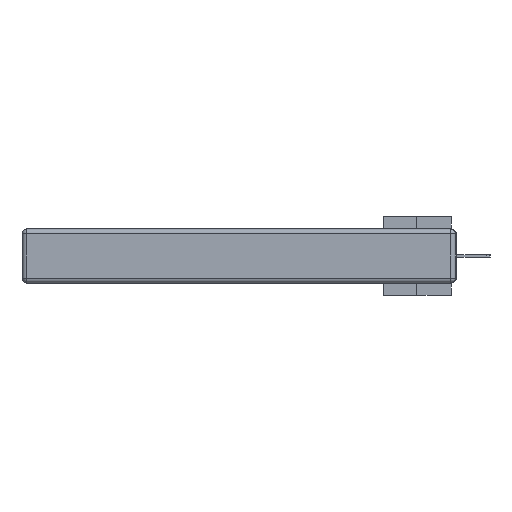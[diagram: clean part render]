
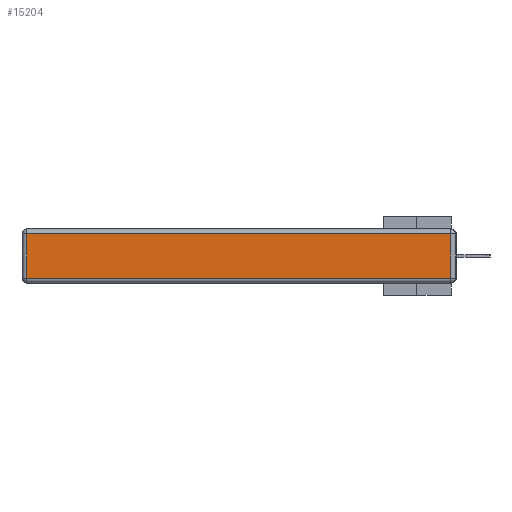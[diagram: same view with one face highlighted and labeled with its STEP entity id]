
A CAD part, left-side view. The second image highlights one B-rep face of the part: STEP entity #15204.
In plain terms, the highlighted planar face has unit normal (-1, 0, 0).
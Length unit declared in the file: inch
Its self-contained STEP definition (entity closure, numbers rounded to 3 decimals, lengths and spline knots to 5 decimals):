
#1295 = DIRECTION ( 'NONE',  ( 0., 0., 1. ) ) ;
#2085 = EDGE_CURVE ( 'NONE', #8228, #25494, #31816, .T. ) ;
#2964 = EDGE_LOOP ( 'NONE', ( #28196, #27298, #23899, #24399 ) ) ;
#3257 = EDGE_CURVE ( 'NONE', #29479, #37648, #40061, .T. ) ;
#3329 = EDGE_CURVE ( 'NONE', #37648, #8228, #33563, .T. ) ;
#4023 = DIRECTION ( 'NONE',  ( 0., 1., 0. ) ) ;
#6081 = EDGE_CURVE ( 'NONE', #25494, #29479, #33803, .T. ) ;
#7036 = VECTOR ( 'NONE', #8781, 39.37008 ) ;
#8228 = VERTEX_POINT ( 'NONE', #17360 ) ;
#8781 = DIRECTION ( 'NONE',  ( 0., 0., -1. ) ) ;
#9344 = VECTOR ( 'NONE', #4023, 39.37008 ) ;
#14401 = DIRECTION ( 'NONE',  ( 0., 0., 1. ) ) ;
#14841 = AXIS2_PLACEMENT_3D ( 'NONE', #17502, #24609, #1295 ) ;
#15038 = CARTESIAN_POINT ( 'NONE',  ( 0., 2.72, -0.343 ) ) ;
#15204 = ADVANCED_FACE ( 'NONE', ( #24806 ), #34475, .T. ) ;
#17360 = CARTESIAN_POINT ( 'NONE',  ( 0., 2.72, -0.03 ) ) ;
#17502 = CARTESIAN_POINT ( 'NONE',  ( 0., 0., -0.343 ) ) ;
#21053 = VECTOR ( 'NONE', #14401, 39.37008 ) ;
#22608 = CARTESIAN_POINT ( 'NONE',  ( 0., 0.03, -0.313 ) ) ;
#23899 = ORIENTED_EDGE ( 'NONE', *, *, #3329, .T. ) ;
#24399 = ORIENTED_EDGE ( 'NONE', *, *, #2085, .T. ) ;
#24609 = DIRECTION ( 'NONE',  ( -1., 0., 0. ) ) ;
#24806 = FACE_OUTER_BOUND ( 'NONE', #2964, .T. ) ;
#25494 = VERTEX_POINT ( 'NONE', #38235 ) ;
#25695 = VECTOR ( 'NONE', #34245, 39.37008 ) ;
#27298 = ORIENTED_EDGE ( 'NONE', *, *, #3257, .T. ) ;
#28196 = ORIENTED_EDGE ( 'NONE', *, *, #6081, .T. ) ;
#29479 = VERTEX_POINT ( 'NONE', #22608 ) ;
#30806 = CARTESIAN_POINT ( 'NONE',  ( 0., 0., -0.313 ) ) ;
#31816 = LINE ( 'NONE', #15038, #7036 ) ;
#33563 = LINE ( 'NONE', #33757, #9344 ) ;
#33757 = CARTESIAN_POINT ( 'NONE',  ( 0., 2.75, -0.03 ) ) ;
#33803 = LINE ( 'NONE', #30806, #25695 ) ;
#34245 = DIRECTION ( 'NONE',  ( 0., -1., 0. ) ) ;
#34475 = PLANE ( 'NONE',  #14841 ) ;
#37648 = VERTEX_POINT ( 'NONE', #40171 ) ;
#38235 = CARTESIAN_POINT ( 'NONE',  ( 0., 2.72, -0.313 ) ) ;
#40061 = LINE ( 'NONE', #40922, #21053 ) ;
#40171 = CARTESIAN_POINT ( 'NONE',  ( 0., 0.03, -0.03 ) ) ;
#40922 = CARTESIAN_POINT ( 'NONE',  ( 0., 0.03, -0.343 ) ) ;
